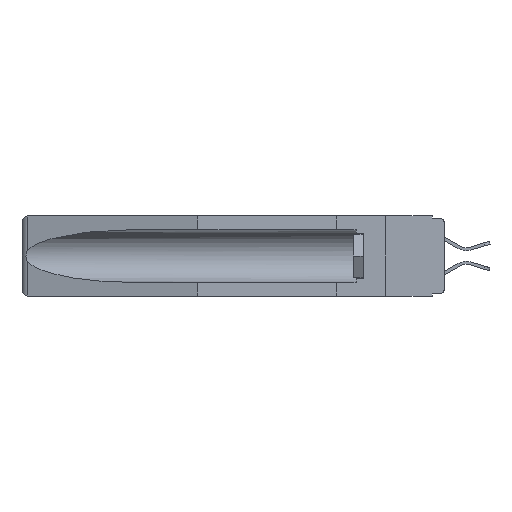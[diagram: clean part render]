
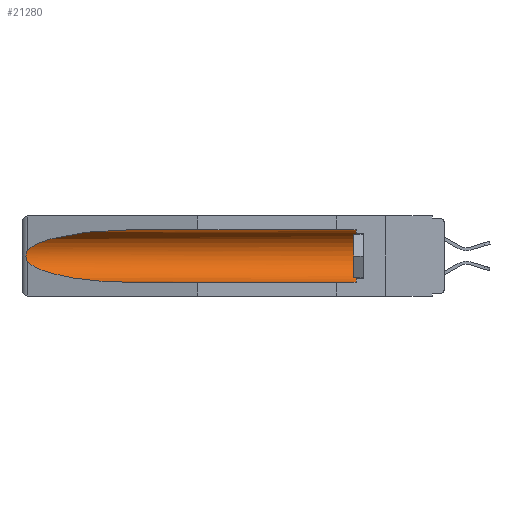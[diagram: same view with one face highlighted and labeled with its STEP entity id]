
A CAD part, left-side view. The second image highlights one B-rep face of the part: STEP entity #21280.
In plain terms, the highlighted cylindrical face has radius 2.857 mm (diameter 5.715 mm), a partial arc.
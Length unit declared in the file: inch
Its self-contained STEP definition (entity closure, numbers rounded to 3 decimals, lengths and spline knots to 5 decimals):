
#79 = CARTESIAN_POINT ( 'NONE',  ( 0.25451, 1.48313, -0.09465 ) ) ;
#304 = CARTESIAN_POINT ( 'NONE',  ( 0.155, 0.126, -0.1715 ) ) ;
#628 = DIRECTION ( 'NONE',  ( 0., 1., 0. ) ) ;
#946 = EDGE_LOOP ( 'NONE', ( #4091, #24211, #12822, #23270, #8658, #23643 ) ) ;
#1376 = CARTESIAN_POINT ( 'NONE',  ( 0.26537, 1.52718, -0.19328 ) ) ;
#2109 = FACE_OUTER_BOUND ( 'NONE', #946, .T. ) ;
#2406 = CARTESIAN_POINT ( 'NONE',  ( 0.26537, 1.52718, -0.14972 ) ) ;
#3171 = DIRECTION ( 'NONE',  ( 0., 0., 1. ) ) ;
#4035 = CARTESIAN_POINT ( 'NONE',  ( 0.2673, 1.53269, -0.17917 ) ) ;
#4091 = ORIENTED_EDGE ( 'NONE', *, *, #20015, .T. ) ;
#4241 = CARTESIAN_POINT ( 'NONE',  ( 0.26537, 1.52718, -0.14972 ) ) ;
#4557 = CARTESIAN_POINT ( 'NONE',  ( 0.26597, 1.5296, -0.19026 ) ) ;
#4645 = CARTESIAN_POINT ( 'NONE',  ( 0.26537, 1.52718, -0.19328 ) ) ;
#5400 = CARTESIAN_POINT ( 'NONE',  ( 0.26537, 1.52718, -0.19328 ) ) ;
#5889 = CARTESIAN_POINT ( 'NONE',  ( 0.26537, 1.52718, -0.14972 ) ) ;
#6390 = CARTESIAN_POINT ( 'NONE',  ( 0.155, -0.30754, -0.059 ) ) ;
#6455 = CARTESIAN_POINT ( 'NONE',  ( 0.155, 1.07973, -0.284 ) ) ;
#7380 = CARTESIAN_POINT ( 'NONE',  ( 0.155, 1.07973, -0.284 ) ) ;
#7937 = CARTESIAN_POINT ( 'NONE',  ( 0.2673, 1.5327, -0.16383 ) ) ;
#8094 = AXIS2_PLACEMENT_3D ( 'NONE', #304, #12579, #10848 ) ;
#8208 = VERTEX_POINT ( 'NONE', #19585 ) ;
#8476 = CYLINDRICAL_SURFACE ( 'NONE', #20588, 0.1125 ) ;
#8658 = ORIENTED_EDGE ( 'NONE', *, *, #13196, .T. ) ;
#8795 = EDGE_CURVE ( 'NONE', #24772, #22781, #19219, .T. ) ;
#8944 = VERTEX_POINT ( 'NONE', #8966 ) ;
#8966 = CARTESIAN_POINT ( 'NONE',  ( 0.155, 0.126, -0.059 ) ) ;
#9400 = CARTESIAN_POINT ( 'NONE',  ( 0.25451, 1.48313, -0.24835 ) ) ;
#9839 = CARTESIAN_POINT ( 'NONE',  ( 0.155, 1.07973, -0.059 ) ) ;
#10187 =( BOUNDED_CURVE ( )  B_SPLINE_CURVE ( 3, ( #5400, #9400, #19769, #7380 ),
 .UNSPECIFIED., .F., .F. ) 
 B_SPLINE_CURVE_WITH_KNOTS ( ( 4, 4 ),
 ( 0.1948, 1.5708 ),
 .UNSPECIFIED. ) 
 CURVE ( )  GEOMETRIC_REPRESENTATION_ITEM ( )  RATIONAL_B_SPLINE_CURVE ( ( 1., 0.848, 0.848, 1. ) ) 
 REPRESENTATION_ITEM ( '' )  );
#10230 = CIRCLE ( 'NONE', #8094, 0.1125 ) ;
#10418 = CARTESIAN_POINT ( 'NONE',  ( 0.21114, 1.30732, -0.059 ) ) ;
#10848 = DIRECTION ( 'NONE',  ( 0., 0., 1. ) ) ;
#11962 = CARTESIAN_POINT ( 'NONE',  ( 0.26597, 1.52961, -0.15275 ) ) ;
#12393 = EDGE_CURVE ( 'NONE', #8944, #24617, #25104, .T. ) ;
#12579 = DIRECTION ( 'NONE',  ( 0., -1., 0. ) ) ;
#12730 = CARTESIAN_POINT ( 'NONE',  ( 0.155, -0.30754, -0.284 ) ) ;
#12822 = ORIENTED_EDGE ( 'NONE', *, *, #18880, .T. ) ;
#13196 = EDGE_CURVE ( 'NONE', #8208, #8944, #10230, .T. ) ;
#14453 = VERTEX_POINT ( 'NONE', #6455 ) ;
#14534 =( BOUNDED_CURVE ( )  B_SPLINE_CURVE ( 3, ( #18169, #10418, #79, #4241 ),
 .UNSPECIFIED., .F., .F. ) 
 B_SPLINE_CURVE_WITH_KNOTS ( ( 4, 4 ),
 ( 4.71239, 6.08839 ),
 .UNSPECIFIED. ) 
 CURVE ( )  GEOMETRIC_REPRESENTATION_ITEM ( )  RATIONAL_B_SPLINE_CURVE ( ( 1., 0.848, 0.848, 1. ) ) 
 REPRESENTATION_ITEM ( '' )  );
#16705 = EDGE_CURVE ( 'NONE', #8208, #14453, #17001, .T. ) ;
#17001 = LINE ( 'NONE', #12730, #23009 ) ;
#18123 = CARTESIAN_POINT ( 'NONE',  ( 0.26655, 1.53094, -0.18657 ) ) ;
#18169 = CARTESIAN_POINT ( 'NONE',  ( 0.155, 1.07973, -0.059 ) ) ;
#18880 = EDGE_CURVE ( 'NONE', #22781, #14453, #10187, .T. ) ;
#19219 = B_SPLINE_CURVE_WITH_KNOTS ( 'NONE', 3,
 ( #5889, #11962, #19978, #7937, #22028, #26061, #4035, #18123, #4557, #4645 ),
 .UNSPECIFIED., .F., .F.,
 ( 4, 2, 2, 2, 4 ),
 ( 0., 0.00029, 0.00058, 0.00087, 0.00117 ),
 .UNSPECIFIED. ) ;
#19387 = CARTESIAN_POINT ( 'NONE',  ( 0.155, -0.30754, -0.1715 ) ) ;
#19585 = CARTESIAN_POINT ( 'NONE',  ( 0.155, 0.126, -0.284 ) ) ;
#19769 = CARTESIAN_POINT ( 'NONE',  ( 0.21114, 1.30732, -0.284 ) ) ;
#19978 = CARTESIAN_POINT ( 'NONE',  ( 0.26654, 1.53092, -0.15636 ) ) ;
#20015 = EDGE_CURVE ( 'NONE', #24617, #24772, #14534, .T. ) ;
#20588 = AXIS2_PLACEMENT_3D ( 'NONE', #19387, #21409, #3171 ) ;
#21280 = ADVANCED_FACE ( 'NONE', ( #2109 ), #8476, .F. ) ;
#21409 = DIRECTION ( 'NONE',  ( 0., 1., 0. ) ) ;
#22028 = CARTESIAN_POINT ( 'NONE',  ( 0.2675, 1.53308, -0.16763 ) ) ;
#22781 = VERTEX_POINT ( 'NONE', #1376 ) ;
#23009 = VECTOR ( 'NONE', #628, 39.37008 ) ;
#23036 = DIRECTION ( 'NONE',  ( 0., 1., 0. ) ) ;
#23270 = ORIENTED_EDGE ( 'NONE', *, *, #16705, .F. ) ;
#23643 = ORIENTED_EDGE ( 'NONE', *, *, #12393, .T. ) ;
#24211 = ORIENTED_EDGE ( 'NONE', *, *, #8795, .T. ) ;
#24452 = VECTOR ( 'NONE', #23036, 39.37008 ) ;
#24617 = VERTEX_POINT ( 'NONE', #9839 ) ;
#24772 = VERTEX_POINT ( 'NONE', #2406 ) ;
#25104 = LINE ( 'NONE', #6390, #24452 ) ;
#26061 = CARTESIAN_POINT ( 'NONE',  ( 0.2675, 1.53308, -0.17534 ) ) ;
